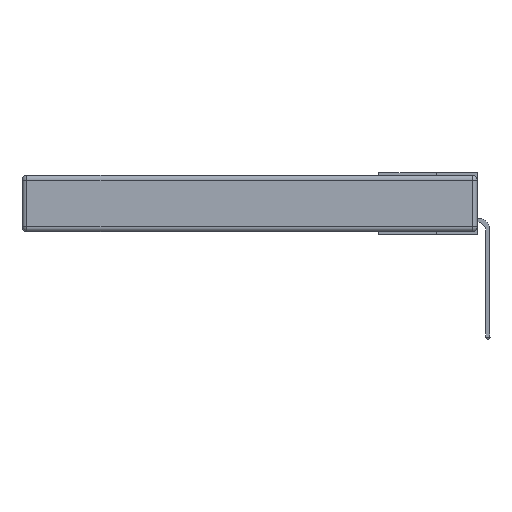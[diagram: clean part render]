
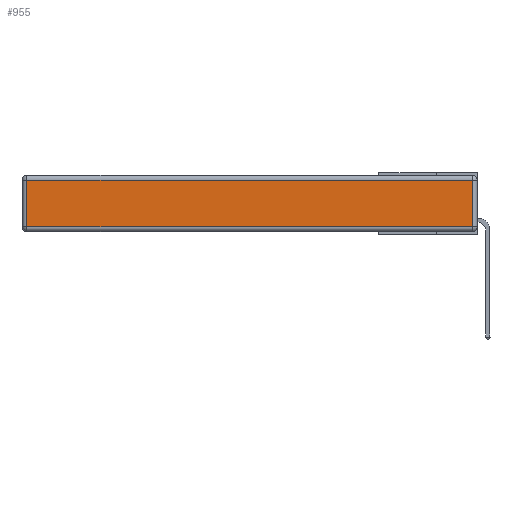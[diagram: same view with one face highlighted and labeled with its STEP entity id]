
A CAD part, left-side view. The second image highlights one B-rep face of the part: STEP entity #955.
In plain terms, the highlighted planar face has unit normal (-1, 0, 0).
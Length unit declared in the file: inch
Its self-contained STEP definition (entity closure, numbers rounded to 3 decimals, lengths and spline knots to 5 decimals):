
#700 = EDGE_CURVE ( 'NONE', #32214, #9722, #18845, .T. ) ;
#955 = ADVANCED_FACE ( 'NONE', ( #23827 ), #20171, .T. ) ;
#1681 = VECTOR ( 'NONE', #19361, 39.37008 ) ;
#1724 = ORIENTED_EDGE ( 'NONE', *, *, #5033, .T. ) ;
#2411 = EDGE_CURVE ( 'NONE', #24130, #31244, #21205, .T. ) ;
#2556 = CARTESIAN_POINT ( 'NONE',  ( 0., 0.03, -0.343 ) ) ;
#4307 = DIRECTION ( 'NONE',  ( 0., 0., 1. ) ) ;
#5033 = EDGE_CURVE ( 'NONE', #9722, #24130, #24727, .T. ) ;
#5440 = CARTESIAN_POINT ( 'NONE',  ( 0., 2.72, -0.313 ) ) ;
#8323 = EDGE_LOOP ( 'NONE', ( #17841, #1724, #17679, #11346 ) ) ;
#9364 = DIRECTION ( 'NONE',  ( 0., 0., 1. ) ) ;
#9722 = VERTEX_POINT ( 'NONE', #21405 ) ;
#9907 = CARTESIAN_POINT ( 'NONE',  ( 0., 2.72, -0.343 ) ) ;
#11346 = ORIENTED_EDGE ( 'NONE', *, *, #14223, .T. ) ;
#11367 = AXIS2_PLACEMENT_3D ( 'NONE', #30697, #22979, #4307 ) ;
#12496 = VECTOR ( 'NONE', #28060, 39.37008 ) ;
#14223 = EDGE_CURVE ( 'NONE', #31244, #32214, #31876, .T. ) ;
#17679 = ORIENTED_EDGE ( 'NONE', *, *, #2411, .T. ) ;
#17841 = ORIENTED_EDGE ( 'NONE', *, *, #700, .T. ) ;
#18244 = CARTESIAN_POINT ( 'NONE',  ( 0., 2.72, -0.03 ) ) ;
#18845 = LINE ( 'NONE', #24259, #1681 ) ;
#18989 = CARTESIAN_POINT ( 'NONE',  ( 0., 0.03, -0.03 ) ) ;
#19361 = DIRECTION ( 'NONE',  ( 0., -1., 0. ) ) ;
#20171 = PLANE ( 'NONE',  #11367 ) ;
#21205 = LINE ( 'NONE', #27945, #12496 ) ;
#21405 = CARTESIAN_POINT ( 'NONE',  ( 0., 0.03, -0.313 ) ) ;
#21847 = VECTOR ( 'NONE', #31466, 39.37008 ) ;
#22979 = DIRECTION ( 'NONE',  ( -1., 0., 0. ) ) ;
#23827 = FACE_OUTER_BOUND ( 'NONE', #8323, .T. ) ;
#24130 = VERTEX_POINT ( 'NONE', #18989 ) ;
#24259 = CARTESIAN_POINT ( 'NONE',  ( 0., 0., -0.313 ) ) ;
#24727 = LINE ( 'NONE', #2556, #34282 ) ;
#27945 = CARTESIAN_POINT ( 'NONE',  ( 0., 2.75, -0.03 ) ) ;
#28060 = DIRECTION ( 'NONE',  ( 0., 1., 0. ) ) ;
#30697 = CARTESIAN_POINT ( 'NONE',  ( 0., 0., -0.343 ) ) ;
#31244 = VERTEX_POINT ( 'NONE', #18244 ) ;
#31466 = DIRECTION ( 'NONE',  ( 0., 0., -1. ) ) ;
#31876 = LINE ( 'NONE', #9907, #21847 ) ;
#32214 = VERTEX_POINT ( 'NONE', #5440 ) ;
#34282 = VECTOR ( 'NONE', #9364, 39.37008 ) ;
